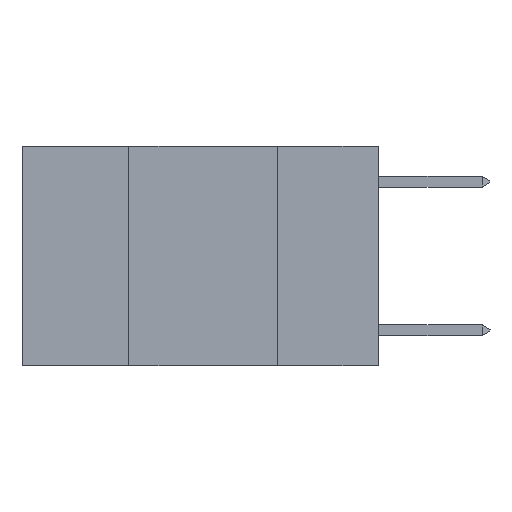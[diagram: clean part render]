
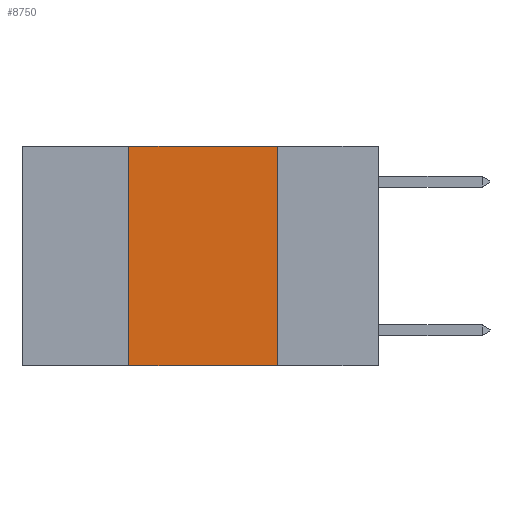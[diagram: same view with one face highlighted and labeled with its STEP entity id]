
A CAD part, left-side view. The second image highlights one B-rep face of the part: STEP entity #8750.
In plain terms, the highlighted planar face has unit normal (-1, 0, 0).
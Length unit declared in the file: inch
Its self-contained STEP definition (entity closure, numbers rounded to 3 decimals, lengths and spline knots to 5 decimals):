
#467 = LINE ( 'NONE', #4535, #3166 ) ;
#2375 = LINE ( 'NONE', #8568, #8975 ) ;
#3166 = VECTOR ( 'NONE', #8455, 39.37008 ) ;
#3702 = CARTESIAN_POINT ( 'NONE',  ( 0., 0.6, -0.37 ) ) ;
#4047 = CARTESIAN_POINT ( 'NONE',  ( 0., 0.42, 0. ) ) ;
#4535 = CARTESIAN_POINT ( 'NONE',  ( 0., 0.6, 0. ) ) ;
#4975 = ORIENTED_EDGE ( 'NONE', *, *, #13926, .F. ) ;
#5475 = ORIENTED_EDGE ( 'NONE', *, *, #12212, .T. ) ;
#5858 = ORIENTED_EDGE ( 'NONE', *, *, #13063, .F. ) ;
#6612 = CARTESIAN_POINT ( 'NONE',  ( 0., 0.17, -0.37 ) ) ;
#6796 = VECTOR ( 'NONE', #9232, 39.37008 ) ;
#8336 = CARTESIAN_POINT ( 'NONE',  ( 0., 0.42, 0. ) ) ;
#8368 = VERTEX_POINT ( 'NONE', #15766 ) ;
#8455 = DIRECTION ( 'NONE',  ( 0., -1., 0. ) ) ;
#8568 = CARTESIAN_POINT ( 'NONE',  ( 0., 0.17, 0. ) ) ;
#8750 = ADVANCED_FACE ( 'NONE', ( #12633 ), #12527, .F. ) ;
#8782 = ORIENTED_EDGE ( 'NONE', *, *, #15825, .F. ) ;
#8897 = VERTEX_POINT ( 'NONE', #11499 ) ;
#8975 = VECTOR ( 'NONE', #9882, 39.37008 ) ;
#9005 = AXIS2_PLACEMENT_3D ( 'NONE', #12579, #12510, #12507 ) ;
#9232 = DIRECTION ( 'NONE',  ( 0., 0., 1. ) ) ;
#9882 = DIRECTION ( 'NONE',  ( 0., 0., -1. ) ) ;
#10250 = LINE ( 'NONE', #4047, #6796 ) ;
#11077 = VERTEX_POINT ( 'NONE', #6612 ) ;
#11499 = CARTESIAN_POINT ( 'NONE',  ( 0., 0.17, 0. ) ) ;
#11569 = DIRECTION ( 'NONE',  ( 0., -1., 0. ) ) ;
#12212 = EDGE_CURVE ( 'NONE', #8368, #11077, #16075, .T. ) ;
#12507 = DIRECTION ( 'NONE',  ( 0., 0., -1. ) ) ;
#12510 = DIRECTION ( 'NONE',  ( 1., 0., 0. ) ) ;
#12527 = PLANE ( 'NONE',  #9005 ) ;
#12579 = CARTESIAN_POINT ( 'NONE',  ( 0., 0.6, 0. ) ) ;
#12633 = FACE_OUTER_BOUND ( 'NONE', #15075, .T. ) ;
#13063 = EDGE_CURVE ( 'NONE', #8368, #13237, #10250, .T. ) ;
#13237 = VERTEX_POINT ( 'NONE', #8336 ) ;
#13926 = EDGE_CURVE ( 'NONE', #8897, #11077, #2375, .T. ) ;
#15075 = EDGE_LOOP ( 'NONE', ( #4975, #8782, #5858, #5475 ) ) ;
#15690 = VECTOR ( 'NONE', #11569, 39.37008 ) ;
#15766 = CARTESIAN_POINT ( 'NONE',  ( 0., 0.42, -0.37 ) ) ;
#15825 = EDGE_CURVE ( 'NONE', #13237, #8897, #467, .T. ) ;
#16075 = LINE ( 'NONE', #3702, #15690 ) ;
